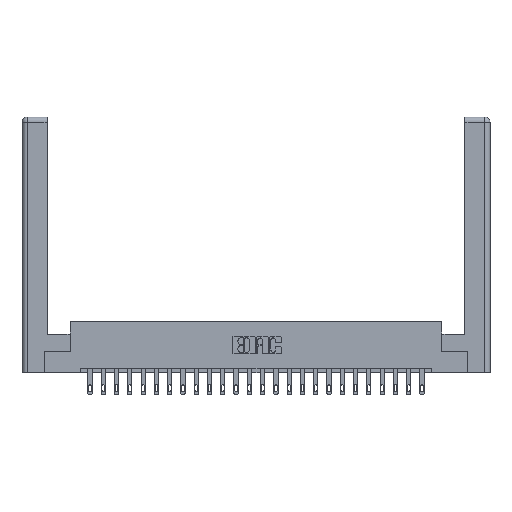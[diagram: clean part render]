
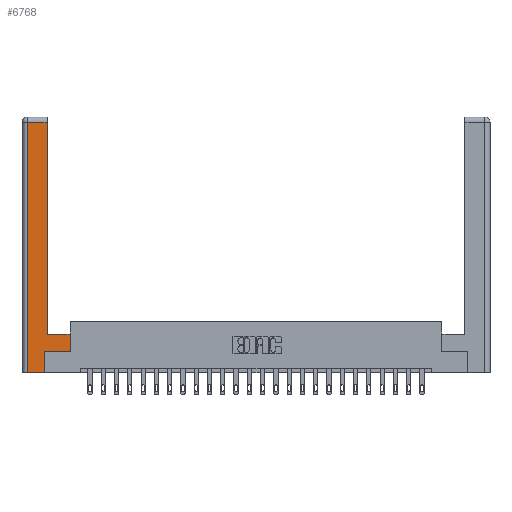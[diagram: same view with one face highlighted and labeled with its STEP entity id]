
A CAD part, top view. The second image highlights one B-rep face of the part: STEP entity #6768.
In plain terms, the highlighted planar face has unit normal (0, 0, 1).
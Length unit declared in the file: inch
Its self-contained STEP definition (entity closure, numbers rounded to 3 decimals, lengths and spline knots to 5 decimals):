
#111 = VERTEX_POINT ( 'NONE', #5250 ) ;
#774 = LINE ( 'NONE', #12250, #23234 ) ;
#1181 = ORIENTED_EDGE ( 'NONE', *, *, #7646, .T. ) ;
#1552 = LINE ( 'NONE', #11799, #9921 ) ;
#1566 = ORIENTED_EDGE ( 'NONE', *, *, #24631, .T. ) ;
#1709 = LINE ( 'NONE', #15554, #16677 ) ;
#1939 = DIRECTION ( 'NONE',  ( -1., 0., 0. ) ) ;
#2246 = ORIENTED_EDGE ( 'NONE', *, *, #7577, .T. ) ;
#2296 = ORIENTED_EDGE ( 'NONE', *, *, #5500, .T. ) ;
#3063 = LINE ( 'NONE', #21503, #21899 ) ;
#4046 = DIRECTION ( 'NONE',  ( 0., 1., 0. ) ) ;
#4432 = DIRECTION ( 'NONE',  ( -1., 0., 0. ) ) ;
#5250 = CARTESIAN_POINT ( 'NONE',  ( 0.565, 0.45, 0. ) ) ;
#5500 = EDGE_CURVE ( 'NONE', #16988, #111, #16365, .T. ) ;
#6072 = DIRECTION ( 'NONE',  ( 0., 1., 0. ) ) ;
#6751 = CARTESIAN_POINT ( 'NONE',  ( 0.565, 0.45, 0. ) ) ;
#6768 = ADVANCED_FACE ( 'NONE', ( #21401 ), #20370, .F. ) ;
#7577 = EDGE_CURVE ( 'NONE', #24135, #20662, #3063, .T. ) ;
#7646 = EDGE_CURVE ( 'NONE', #10961, #16988, #18249, .T. ) ;
#7748 = EDGE_LOOP ( 'NONE', ( #2246, #21321, #18353, #13746, #1566, #1181, #2296, #24153 ) ) ;
#8369 = VECTOR ( 'NONE', #4046, 39.37008 ) ;
#9221 = CARTESIAN_POINT ( 'NONE',  ( 0.265, 0., 0. ) ) ;
#9533 = CARTESIAN_POINT ( 'NONE',  ( 0.0615, 0., 0. ) ) ;
#9921 = VECTOR ( 'NONE', #12043, 39.37008 ) ;
#9960 = CARTESIAN_POINT ( 'NONE',  ( 0.565, 0.245, 0. ) ) ;
#10961 = VERTEX_POINT ( 'NONE', #13589 ) ;
#11313 = VECTOR ( 'NONE', #22356, 39.37008 ) ;
#11799 = CARTESIAN_POINT ( 'NONE',  ( 0.295, 0.45, 0. ) ) ;
#12043 = DIRECTION ( 'NONE',  ( -1., 0., 0. ) ) ;
#12088 = DIRECTION ( 'NONE',  ( 1., 0., 0. ) ) ;
#12250 = CARTESIAN_POINT ( 'NONE',  ( 0.0615, 0., 0. ) ) ;
#12336 = DIRECTION ( 'NONE',  ( 0., -1., 0. ) ) ;
#13589 = CARTESIAN_POINT ( 'NONE',  ( 0.265, 0.245, 0. ) ) ;
#13629 = DIRECTION ( 'NONE',  ( 1., 0., 0. ) ) ;
#13746 = ORIENTED_EDGE ( 'NONE', *, *, #24721, .T. ) ;
#13896 = VERTEX_POINT ( 'NONE', #9221 ) ;
#14642 = VECTOR ( 'NONE', #12088, 39.37008 ) ;
#15554 = CARTESIAN_POINT ( 'NONE',  ( 0.0615, 2.94, 0. ) ) ;
#15618 = VECTOR ( 'NONE', #13629, 39.37008 ) ;
#16290 = CARTESIAN_POINT ( 'NONE',  ( 0.295, 0.45, 0. ) ) ;
#16365 = LINE ( 'NONE', #6751, #11313 ) ;
#16677 = VECTOR ( 'NONE', #4432, 39.37008 ) ;
#16859 = DIRECTION ( 'NONE',  ( 0., 0., -1. ) ) ;
#16988 = VERTEX_POINT ( 'NONE', #17110 ) ;
#17110 = CARTESIAN_POINT ( 'NONE',  ( 0.565, 0.245, 0. ) ) ;
#17417 = CARTESIAN_POINT ( 'NONE',  ( 0.265, 0.245, 0. ) ) ;
#18150 = EDGE_CURVE ( 'NONE', #20662, #24457, #1709, .T. ) ;
#18249 = LINE ( 'NONE', #9960, #15618 ) ;
#18353 = ORIENTED_EDGE ( 'NONE', *, *, #19429, .T. ) ;
#19429 = EDGE_CURVE ( 'NONE', #24457, #23731, #774, .T. ) ;
#20370 = PLANE ( 'NONE',  #22086 ) ;
#20662 = VERTEX_POINT ( 'NONE', #23476 ) ;
#20911 = LINE ( 'NONE', #23845, #14642 ) ;
#21321 = ORIENTED_EDGE ( 'NONE', *, *, #18150, .T. ) ;
#21401 = FACE_OUTER_BOUND ( 'NONE', #7748, .T. ) ;
#21503 = CARTESIAN_POINT ( 'NONE',  ( 0.295, 3., 0. ) ) ;
#21899 = VECTOR ( 'NONE', #6072, 39.37008 ) ;
#22039 = EDGE_CURVE ( 'NONE', #111, #24135, #1552, .T. ) ;
#22086 = AXIS2_PLACEMENT_3D ( 'NONE', #24240, #16859, #1939 ) ;
#22356 = DIRECTION ( 'NONE',  ( 0., 1., 0. ) ) ;
#23234 = VECTOR ( 'NONE', #12336, 39.37008 ) ;
#23308 = LINE ( 'NONE', #17417, #8369 ) ;
#23476 = CARTESIAN_POINT ( 'NONE',  ( 0.295, 2.94, 0. ) ) ;
#23731 = VERTEX_POINT ( 'NONE', #9533 ) ;
#23845 = CARTESIAN_POINT ( 'NONE',  ( 0.265, 0., 0. ) ) ;
#24135 = VERTEX_POINT ( 'NONE', #16290 ) ;
#24153 = ORIENTED_EDGE ( 'NONE', *, *, #22039, .T. ) ;
#24240 = CARTESIAN_POINT ( 'NONE',  ( 0., 0., 0. ) ) ;
#24345 = CARTESIAN_POINT ( 'NONE',  ( 0.0615, 2.94, 0. ) ) ;
#24457 = VERTEX_POINT ( 'NONE', #24345 ) ;
#24631 = EDGE_CURVE ( 'NONE', #13896, #10961, #23308, .T. ) ;
#24721 = EDGE_CURVE ( 'NONE', #23731, #13896, #20911, .T. ) ;
